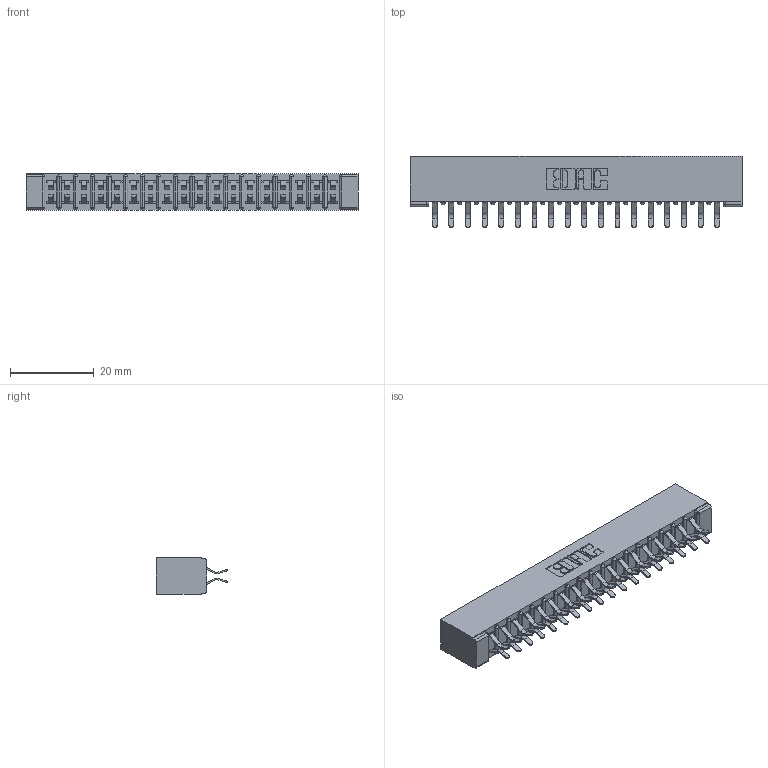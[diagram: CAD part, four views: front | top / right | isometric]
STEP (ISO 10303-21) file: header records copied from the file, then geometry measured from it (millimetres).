
FILE_DESCRIPTION (( 'STEP AP203' ), '1' );
FILE_NAME ('357-036-556-201.STEP', '2018-08-10T06:38:23', ( '' ), ( '' ), 'SwSTEP 2.0', 'SolidWorks 2016', '' );
FILE_SCHEMA (( 'CONFIG_CONTROL_DESIGN' ));
Length unit declared in the file: inch
Products named in the file (3): 307-290-001_556; 357-036-556-201; 307 Part_No Mounting Lugs
Assembly tree (37 placements, depth 2):
  357-036-556-201
    307 Part_No Mounting Lugs
    307-290-001_556  x36
Bounding box: 79.2 x 16.97 x 8.71 mm (x, y, z)
Volume: 5407.4 mm3; surface area: 9776.8 mm2
Topology: 37 solids, 37 shells, 1929 faces, 5411 edges, 3506 vertices
Faces by surface type: plane 1254, cylinder 637, sphere 38
Entity records: 18792 total; most frequent: CARTESIAN_POINT 3078, ORIENTED_EDGE 3046, DIRECTION 3025, EDGE_CURVE 1523, LINE 1159, VECTOR 1159, VERTEX_POINT 986, AXIS2_PLACEMENT_3D 933
